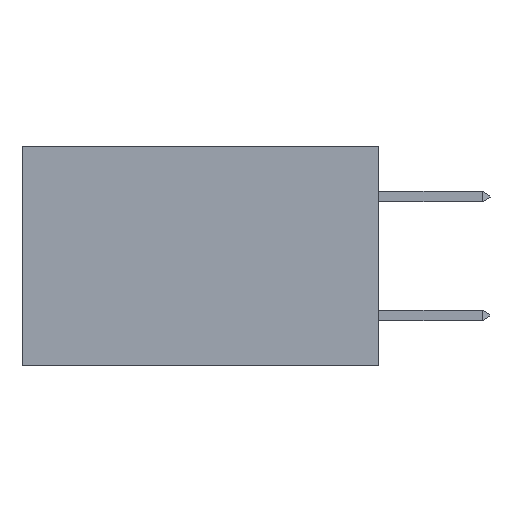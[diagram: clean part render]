
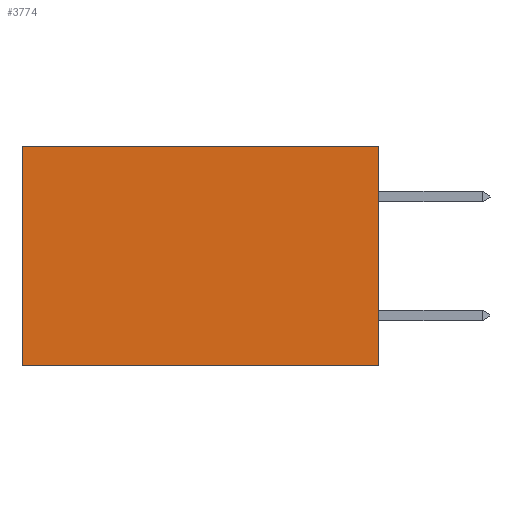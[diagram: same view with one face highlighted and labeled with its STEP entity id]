
A CAD part, left-side view. The second image highlights one B-rep face of the part: STEP entity #3774.
In plain terms, the highlighted planar face has unit normal (-1, 0, 0).
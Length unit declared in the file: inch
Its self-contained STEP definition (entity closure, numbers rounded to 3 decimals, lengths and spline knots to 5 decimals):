
#632 = VERTEX_POINT ( 'NONE', #5287 ) ;
#823 = VERTEX_POINT ( 'NONE', #9767 ) ;
#2190 = VECTOR ( 'NONE', #13769, 39.37008 ) ;
#2564 = ORIENTED_EDGE ( 'NONE', *, *, #20973, .F. ) ;
#2619 = CARTESIAN_POINT ( 'NONE',  ( 0.298, 0., 0. ) ) ;
#3774 = ADVANCED_FACE ( 'NONE', ( #20143 ), #11091, .F. ) ;
#4602 = ORIENTED_EDGE ( 'NONE', *, *, #17555, .T. ) ;
#5101 = DIRECTION ( 'NONE',  ( 0., 0., -1. ) ) ;
#5287 = CARTESIAN_POINT ( 'NONE',  ( 0.298, 0., 0. ) ) ;
#6691 = VECTOR ( 'NONE', #25391, 39.37008 ) ;
#9767 = CARTESIAN_POINT ( 'NONE',  ( 0.298, 0.6, -0.37 ) ) ;
#10901 = DIRECTION ( 'NONE',  ( 1., 0., 0. ) ) ;
#11073 = CARTESIAN_POINT ( 'NONE',  ( 0.298, 0., 0. ) ) ;
#11091 = PLANE ( 'NONE',  #27031 ) ;
#11274 = CARTESIAN_POINT ( 'NONE',  ( 0.298, 0., 0. ) ) ;
#11870 = VECTOR ( 'NONE', #5101, 39.37008 ) ;
#12590 = VERTEX_POINT ( 'NONE', #31226 ) ;
#12675 = LINE ( 'NONE', #24598, #11870 ) ;
#13247 = LINE ( 'NONE', #18042, #6691 ) ;
#13769 = DIRECTION ( 'NONE',  ( 0., 1., 0. ) ) ;
#14481 = EDGE_LOOP ( 'NONE', ( #4602, #2564, #15460, #18746 ) ) ;
#14513 = LINE ( 'NONE', #11073, #27467 ) ;
#15460 = ORIENTED_EDGE ( 'NONE', *, *, #18306, .F. ) ;
#15955 = CARTESIAN_POINT ( 'NONE',  ( 0.298, 0., -0.37 ) ) ;
#16088 = LINE ( 'NONE', #11274, #2190 ) ;
#17555 = EDGE_CURVE ( 'NONE', #12590, #823, #12675, .T. ) ;
#17805 = VERTEX_POINT ( 'NONE', #15955 ) ;
#18042 = CARTESIAN_POINT ( 'NONE',  ( 0.298, 0., -0.37 ) ) ;
#18306 = EDGE_CURVE ( 'NONE', #632, #17805, #14513, .T. ) ;
#18746 = ORIENTED_EDGE ( 'NONE', *, *, #23076, .T. ) ;
#20143 = FACE_OUTER_BOUND ( 'NONE', #14481, .T. ) ;
#20973 = EDGE_CURVE ( 'NONE', #17805, #823, #13247, .T. ) ;
#23076 = EDGE_CURVE ( 'NONE', #632, #12590, #16088, .T. ) ;
#24598 = CARTESIAN_POINT ( 'NONE',  ( 0.298, 0.6, 0. ) ) ;
#25391 = DIRECTION ( 'NONE',  ( 0., 1., 0. ) ) ;
#26001 = DIRECTION ( 'NONE',  ( 0., 0., -1. ) ) ;
#27031 = AXIS2_PLACEMENT_3D ( 'NONE', #2619, #10901, #26001 ) ;
#27467 = VECTOR ( 'NONE', #28164, 39.37008 ) ;
#28164 = DIRECTION ( 'NONE',  ( 0., 0., -1. ) ) ;
#31226 = CARTESIAN_POINT ( 'NONE',  ( 0.298, 0.6, 0. ) ) ;
